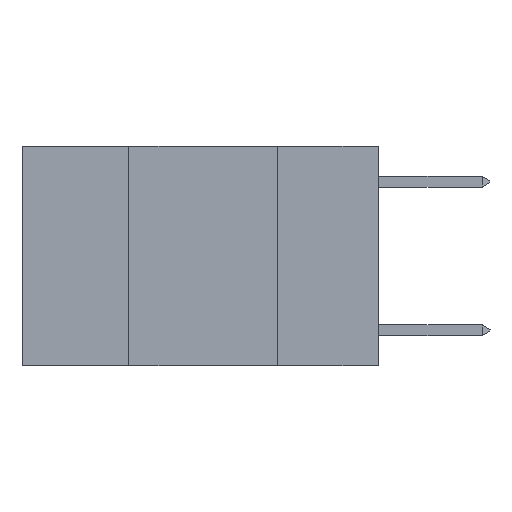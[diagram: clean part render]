
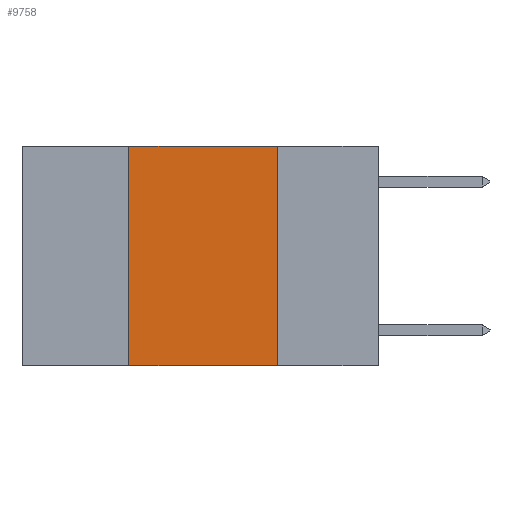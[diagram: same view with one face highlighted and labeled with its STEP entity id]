
A CAD part, left-side view. The second image highlights one B-rep face of the part: STEP entity #9758.
In plain terms, the highlighted planar face has unit normal (-1, 0, 0).
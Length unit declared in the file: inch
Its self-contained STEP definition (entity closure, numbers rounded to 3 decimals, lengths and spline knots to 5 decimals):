
#201 = DIRECTION ( 'NONE',  ( 0., -1., 0. ) ) ;
#417 = CARTESIAN_POINT ( 'NONE',  ( 0., 0.6, -0.37 ) ) ;
#806 = CARTESIAN_POINT ( 'NONE',  ( 0., 0.17, -0.37 ) ) ;
#899 = VERTEX_POINT ( 'NONE', #8744 ) ;
#1013 = ORIENTED_EDGE ( 'NONE', *, *, #4503, .T. ) ;
#1413 = CARTESIAN_POINT ( 'NONE',  ( 0., 0.42, -0.37 ) ) ;
#2066 = EDGE_CURVE ( 'NONE', #3692, #10335, #7228, .T. ) ;
#2429 = DIRECTION ( 'NONE',  ( 0., 0., -1. ) ) ;
#2452 = DIRECTION ( 'NONE',  ( 1., 0., 0. ) ) ;
#2474 = CARTESIAN_POINT ( 'NONE',  ( 0., 0.6, 0. ) ) ;
#2517 = PLANE ( 'NONE',  #9261 ) ;
#2741 = CARTESIAN_POINT ( 'NONE',  ( 0., 0.42, 0. ) ) ;
#3692 = VERTEX_POINT ( 'NONE', #1413 ) ;
#3871 = ORIENTED_EDGE ( 'NONE', *, *, #2066, .F. ) ;
#4503 = EDGE_CURVE ( 'NONE', #3692, #8623, #6672, .T. ) ;
#4869 = DIRECTION ( 'NONE',  ( 0., -1., 0. ) ) ;
#5630 = EDGE_CURVE ( 'NONE', #10335, #899, #8719, .T. ) ;
#5728 = VECTOR ( 'NONE', #201, 39.37008 ) ;
#5791 = FACE_OUTER_BOUND ( 'NONE', #10632, .T. ) ;
#5811 = EDGE_CURVE ( 'NONE', #899, #8623, #6392, .T. ) ;
#5853 = VECTOR ( 'NONE', #6463, 39.37008 ) ;
#6392 = LINE ( 'NONE', #7344, #5853 ) ;
#6463 = DIRECTION ( 'NONE',  ( 0., 0., -1. ) ) ;
#6672 = LINE ( 'NONE', #417, #5728 ) ;
#7228 = LINE ( 'NONE', #8088, #7323 ) ;
#7323 = VECTOR ( 'NONE', #8010, 39.37008 ) ;
#7344 = CARTESIAN_POINT ( 'NONE',  ( 0., 0.17, 0. ) ) ;
#7802 = ORIENTED_EDGE ( 'NONE', *, *, #5630, .F. ) ;
#8010 = DIRECTION ( 'NONE',  ( 0., 0., 1. ) ) ;
#8088 = CARTESIAN_POINT ( 'NONE',  ( 0., 0.42, 0. ) ) ;
#8466 = VECTOR ( 'NONE', #4869, 39.37008 ) ;
#8623 = VERTEX_POINT ( 'NONE', #806 ) ;
#8659 = ORIENTED_EDGE ( 'NONE', *, *, #5811, .F. ) ;
#8719 = LINE ( 'NONE', #10497, #8466 ) ;
#8744 = CARTESIAN_POINT ( 'NONE',  ( 0., 0.17, 0. ) ) ;
#9261 = AXIS2_PLACEMENT_3D ( 'NONE', #2474, #2452, #2429 ) ;
#9758 = ADVANCED_FACE ( 'NONE', ( #5791 ), #2517, .F. ) ;
#10335 = VERTEX_POINT ( 'NONE', #2741 ) ;
#10497 = CARTESIAN_POINT ( 'NONE',  ( 0., 0.6, 0. ) ) ;
#10632 = EDGE_LOOP ( 'NONE', ( #8659, #7802, #3871, #1013 ) ) ;
